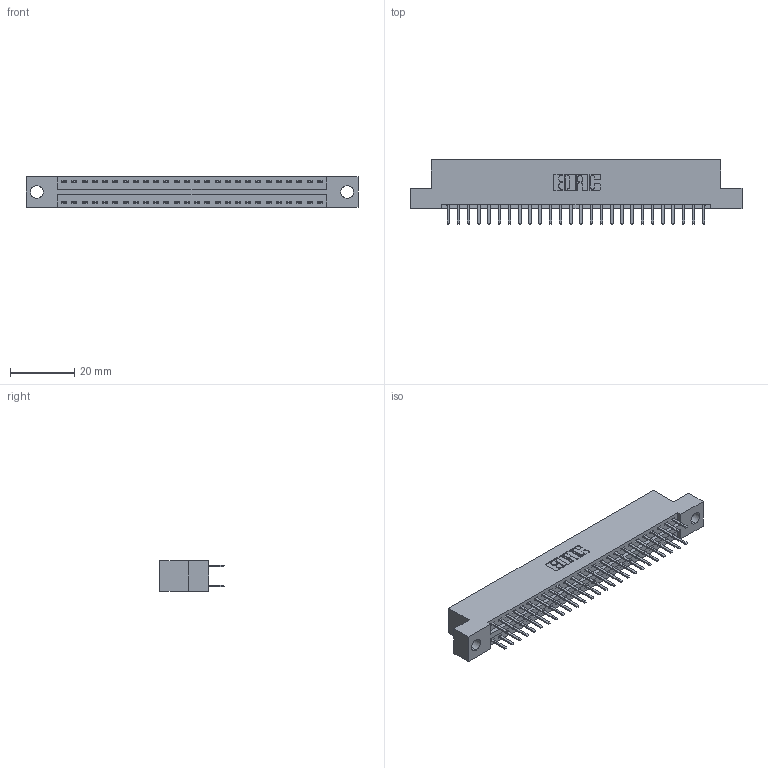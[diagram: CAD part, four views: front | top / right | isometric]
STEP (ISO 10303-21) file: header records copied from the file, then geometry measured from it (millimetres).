
FILE_DESCRIPTION (( 'STEP AP203' ), '1' );
FILE_NAME ('346-052-520-204.STEP', '2022-05-21T00:33:51', ( '' ), ( '' ), 'SwSTEP 2.0', 'SolidWorks 2020', '' );
FILE_SCHEMA (( 'CONFIG_CONTROL_DESIGN' ));
Length unit declared in the file: inch
Products named in the file (3): 346 Part_Flush Mounting Lugs - 0.156 Dia-TH; 346-052-520-204; 345-292-001_345-293-120
Assembly tree (53 placements, depth 2):
  346-052-520-204
    346 Part_Flush Mounting Lugs - 0.156 Dia-TH
    345-292-001_345-293-120  x52
Bounding box: 103.12 x 20.02 x 9.4 mm (x, y, z)
Volume: 9802.8 mm3; surface area: 13017.4 mm2
Topology: 53 solids, 53 shells, 3048 faces, 8841 edges, 5754 vertices
Faces by surface type: plane 2014, cylinder 1034
Entity records: 19655 total; most frequent: CARTESIAN_POINT 3278, ORIENTED_EDGE 3198, DIRECTION 2927, EDGE_CURVE 1599, LINE 1359, VECTOR 1359, VERTEX_POINT 1062, AXIS2_PLACEMENT_3D 784
